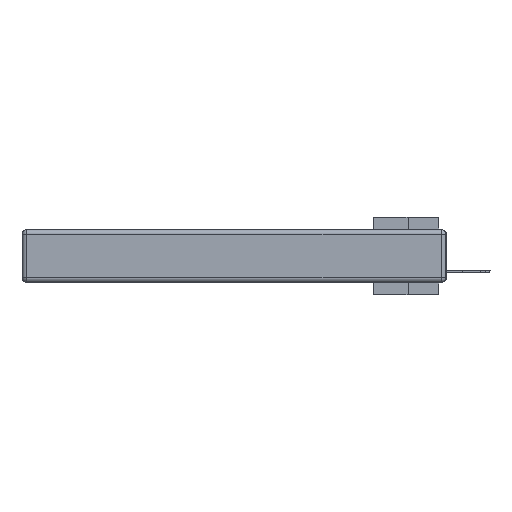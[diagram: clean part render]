
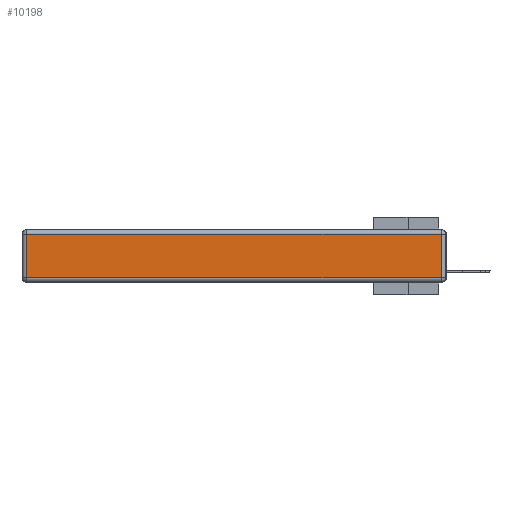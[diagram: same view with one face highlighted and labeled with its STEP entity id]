
A CAD part, left-side view. The second image highlights one B-rep face of the part: STEP entity #10198.
In plain terms, the highlighted planar face has unit normal (-1, 0, 0).
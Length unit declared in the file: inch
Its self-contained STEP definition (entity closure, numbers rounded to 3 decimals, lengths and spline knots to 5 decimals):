
#1831 = VERTEX_POINT ( 'NONE', #16751 ) ;
#2230 = DIRECTION ( 'NONE',  ( 0., 1., 0. ) ) ;
#4135 = PLANE ( 'NONE',  #30596 ) ;
#7112 = LINE ( 'NONE', #28479, #36408 ) ;
#7783 = DIRECTION ( 'NONE',  ( 0., 0., 1. ) ) ;
#8973 = EDGE_CURVE ( 'NONE', #22534, #1831, #14317, .T. ) ;
#10198 = ADVANCED_FACE ( 'NONE', ( #13923 ), #4135, .T. ) ;
#10339 = CARTESIAN_POINT ( 'NONE',  ( 0., 2.72, -0.03 ) ) ;
#10696 = EDGE_LOOP ( 'NONE', ( #14676, #17569, #25522, #37236 ) ) ;
#11012 = DIRECTION ( 'NONE',  ( 0., 0., -1. ) ) ;
#12169 = VERTEX_POINT ( 'NONE', #10339 ) ;
#13923 = FACE_OUTER_BOUND ( 'NONE', #10696, .T. ) ;
#14317 = LINE ( 'NONE', #14534, #17659 ) ;
#14534 = CARTESIAN_POINT ( 'NONE',  ( 0., 0.03, -0.343 ) ) ;
#14676 = ORIENTED_EDGE ( 'NONE', *, *, #24418, .T. ) ;
#15706 = EDGE_CURVE ( 'NONE', #1831, #12169, #36999, .T. ) ;
#16751 = CARTESIAN_POINT ( 'NONE',  ( 0., 0.03, -0.03 ) ) ;
#17450 = VERTEX_POINT ( 'NONE', #26089 ) ;
#17569 = ORIENTED_EDGE ( 'NONE', *, *, #8973, .T. ) ;
#17649 = EDGE_CURVE ( 'NONE', #12169, #17450, #32398, .T. ) ;
#17659 = VECTOR ( 'NONE', #35879, 39.37008 ) ;
#18514 = CARTESIAN_POINT ( 'NONE',  ( 0., 2.75, -0.03 ) ) ;
#22534 = VERTEX_POINT ( 'NONE', #38751 ) ;
#24418 = EDGE_CURVE ( 'NONE', #17450, #22534, #7112, .T. ) ;
#25522 = ORIENTED_EDGE ( 'NONE', *, *, #15706, .T. ) ;
#26089 = CARTESIAN_POINT ( 'NONE',  ( 0., 2.72, -0.313 ) ) ;
#28479 = CARTESIAN_POINT ( 'NONE',  ( 0., 0., -0.313 ) ) ;
#28900 = VECTOR ( 'NONE', #11012, 39.37008 ) ;
#29153 = DIRECTION ( 'NONE',  ( -1., 0., 0. ) ) ;
#30596 = AXIS2_PLACEMENT_3D ( 'NONE', #35684, #29153, #7783 ) ;
#31358 = DIRECTION ( 'NONE',  ( 0., -1., 0. ) ) ;
#32398 = LINE ( 'NONE', #35653, #28900 ) ;
#33487 = VECTOR ( 'NONE', #2230, 39.37008 ) ;
#35653 = CARTESIAN_POINT ( 'NONE',  ( 0., 2.72, -0.343 ) ) ;
#35684 = CARTESIAN_POINT ( 'NONE',  ( 0., 0., -0.343 ) ) ;
#35879 = DIRECTION ( 'NONE',  ( 0., 0., 1. ) ) ;
#36408 = VECTOR ( 'NONE', #31358, 39.37008 ) ;
#36999 = LINE ( 'NONE', #18514, #33487 ) ;
#37236 = ORIENTED_EDGE ( 'NONE', *, *, #17649, .T. ) ;
#38751 = CARTESIAN_POINT ( 'NONE',  ( 0., 0.03, -0.313 ) ) ;
